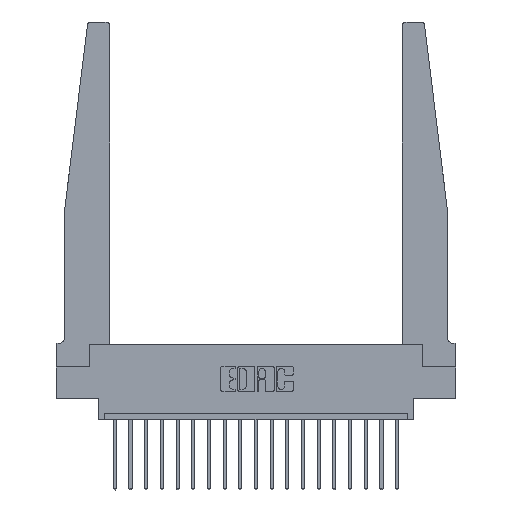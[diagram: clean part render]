
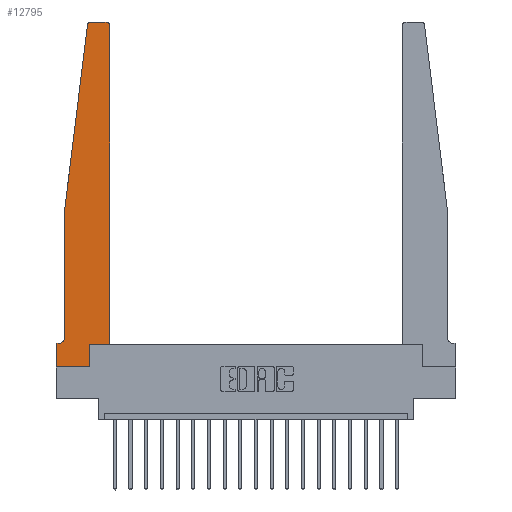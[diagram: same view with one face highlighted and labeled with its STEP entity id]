
A CAD part, top view. The second image highlights one B-rep face of the part: STEP entity #12795.
In plain terms, the highlighted planar face has unit normal (0, 0, 1).
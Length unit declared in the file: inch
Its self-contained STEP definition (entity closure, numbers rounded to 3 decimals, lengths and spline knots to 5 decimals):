
#38 = VECTOR ( 'NONE', #6142, 39.37008 ) ;
#186 = EDGE_CURVE ( 'NONE', #5363, #9330, #9167, .T. ) ;
#230 = EDGE_CURVE ( 'NONE', #16944, #18706, #1505, .T. ) ;
#235 = VECTOR ( 'NONE', #11786, 39.37008 ) ;
#839 = CARTESIAN_POINT ( 'NONE',  ( 0.2605, 0.18, 0.37 ) ) ;
#894 = DIRECTION ( 'NONE',  ( -0.122, -0.992, 0. ) ) ;
#999 = VERTEX_POINT ( 'NONE', #16890 ) ;
#1079 = EDGE_CURVE ( 'NONE', #7324, #6029, #4122, .T. ) ;
#1306 = CARTESIAN_POINT ( 'NONE',  ( 0., 0.1875, 0.37 ) ) ;
#1443 = DIRECTION ( 'NONE',  ( 1., 0., 0. ) ) ;
#1505 = LINE ( 'NONE', #12747, #19449 ) ;
#1701 = AXIS2_PLACEMENT_3D ( 'NONE', #11282, #2000, #12703 ) ;
#2000 = DIRECTION ( 'NONE',  ( 0., 0., -1. ) ) ;
#2064 = CIRCLE ( 'NONE', #1701, 0.05 ) ;
#2297 = CARTESIAN_POINT ( 'NONE',  ( 0.24675, 2.72367, 0.37 ) ) ;
#2537 = CARTESIAN_POINT ( 'NONE',  ( 0.2605, 0., 0.37 ) ) ;
#2604 = LINE ( 'NONE', #17732, #18651 ) ;
#2693 = ORIENTED_EDGE ( 'NONE', *, *, #6544, .T. ) ;
#2717 = VERTEX_POINT ( 'NONE', #5781 ) ;
#2848 = VERTEX_POINT ( 'NONE', #10034 ) ;
#2990 = EDGE_CURVE ( 'NONE', #15976, #16944, #7372, .T. ) ;
#3163 = EDGE_CURVE ( 'NONE', #2717, #12311, #14810, .T. ) ;
#3728 = CARTESIAN_POINT ( 'NONE',  ( 0.27653, 2.72, 0.37 ) ) ;
#3818 = LINE ( 'NONE', #16349, #235 ) ;
#4122 = LINE ( 'NONE', #18320, #38 ) ;
#4577 = PLANE ( 'NONE',  #9474 ) ;
#4659 = VECTOR ( 'NONE', #6564, 39.37008 ) ;
#4793 = CARTESIAN_POINT ( 'NONE',  ( 0.015, 0.1875, 0.37 ) ) ;
#5363 = VERTEX_POINT ( 'NONE', #4793 ) ;
#5781 = CARTESIAN_POINT ( 'NONE',  ( 0., 0., 0.37 ) ) ;
#6029 = VERTEX_POINT ( 'NONE', #18327 ) ;
#6142 = DIRECTION ( 'NONE',  ( 1., 0., 0. ) ) ;
#6544 = EDGE_CURVE ( 'NONE', #18706, #999, #19489, .T. ) ;
#6564 = DIRECTION ( 'NONE',  ( -1., 0., 0. ) ) ;
#6649 = CARTESIAN_POINT ( 'NONE',  ( 0., 0.1875, 0.37 ) ) ;
#6730 = DIRECTION ( 'NONE',  ( 0., 0., 1. ) ) ;
#6944 = CARTESIAN_POINT ( 'NONE',  ( 0.25, 2.75, 0.37 ) ) ;
#7072 = ORIENTED_EDGE ( 'NONE', *, *, #9172, .T. ) ;
#7324 = VERTEX_POINT ( 'NONE', #839 ) ;
#7372 = CIRCLE ( 'NONE', #12401, 0.03 ) ;
#7405 = ORIENTED_EDGE ( 'NONE', *, *, #2990, .T. ) ;
#8124 = DIRECTION ( 'NONE',  ( 1., 0., 0. ) ) ;
#8741 = DIRECTION ( 'NONE',  ( 0., 1., 0. ) ) ;
#9167 = LINE ( 'NONE', #18849, #4659 ) ;
#9172 = EDGE_CURVE ( 'NONE', #2848, #15976, #13660, .T. ) ;
#9330 = VERTEX_POINT ( 'NONE', #6649 ) ;
#9474 = AXIS2_PLACEMENT_3D ( 'NONE', #1306, #12198, #1443 ) ;
#9596 = VECTOR ( 'NONE', #11514, 39.37008 ) ;
#9600 = CARTESIAN_POINT ( 'NONE',  ( 0.395, 2.72, 0.37 ) ) ;
#9708 = AXIS2_PLACEMENT_3D ( 'NONE', #9600, #9785, #11363 ) ;
#9785 = DIRECTION ( 'NONE',  ( 0., 0., 1. ) ) ;
#9899 = CARTESIAN_POINT ( 'NONE',  ( 0.27653, 2.75, 0.37 ) ) ;
#10034 = CARTESIAN_POINT ( 'NONE',  ( 0.395, 2.75, 0.37 ) ) ;
#10244 = VECTOR ( 'NONE', #8124, 39.37008 ) ;
#10257 = ORIENTED_EDGE ( 'NONE', *, *, #18606, .T. ) ;
#10651 = FACE_OUTER_BOUND ( 'NONE', #11011, .T. ) ;
#10748 = EDGE_CURVE ( 'NONE', #9330, #2717, #2604, .T. ) ;
#10983 = VERTEX_POINT ( 'NONE', #14713 ) ;
#11011 = EDGE_LOOP ( 'NONE', ( #7072, #7405, #17081, #2693, #10257, #17054, #12189, #18938, #13365, #11149, #11372, #18903 ) ) ;
#11149 = ORIENTED_EDGE ( 'NONE', *, *, #1079, .T. ) ;
#11225 = CARTESIAN_POINT ( 'NONE',  ( 0., 0., 0.37 ) ) ;
#11282 = CARTESIAN_POINT ( 'NONE',  ( 0.015, 0.2375, 0.37 ) ) ;
#11363 = DIRECTION ( 'NONE',  ( 1., 0., 0. ) ) ;
#11372 = ORIENTED_EDGE ( 'NONE', *, *, #17017, .T. ) ;
#11514 = DIRECTION ( 'NONE',  ( -1., 0., 0. ) ) ;
#11786 = DIRECTION ( 'NONE',  ( 0., 1., 0. ) ) ;
#12189 = ORIENTED_EDGE ( 'NONE', *, *, #10748, .T. ) ;
#12198 = DIRECTION ( 'NONE',  ( 0., 0., 1. ) ) ;
#12311 = VERTEX_POINT ( 'NONE', #2537 ) ;
#12401 = AXIS2_PLACEMENT_3D ( 'NONE', #3728, #6730, #18752 ) ;
#12484 = EDGE_CURVE ( 'NONE', #10983, #2848, #17376, .T. ) ;
#12522 = VECTOR ( 'NONE', #8741, 39.37008 ) ;
#12703 = DIRECTION ( 'NONE',  ( -1., 0., 0. ) ) ;
#12747 = CARTESIAN_POINT ( 'NONE',  ( 0.065, 1.25, 0.37 ) ) ;
#12795 = ADVANCED_FACE ( 'NONE', ( #10651 ), #4577, .T. ) ;
#13365 = ORIENTED_EDGE ( 'NONE', *, *, #13941, .T. ) ;
#13660 = LINE ( 'NONE', #6944, #9596 ) ;
#13941 = EDGE_CURVE ( 'NONE', #12311, #7324, #19233, .T. ) ;
#14713 = CARTESIAN_POINT ( 'NONE',  ( 0.425, 2.72, 0.37 ) ) ;
#14810 = LINE ( 'NONE', #11225, #10244 ) ;
#15223 = CARTESIAN_POINT ( 'NONE',  ( 0.065, 1.25, 0.37 ) ) ;
#15976 = VERTEX_POINT ( 'NONE', #9899 ) ;
#16324 = DIRECTION ( 'NONE',  ( 0., -1., 0. ) ) ;
#16349 = CARTESIAN_POINT ( 'NONE',  ( 0.425, 0.18, 0.37 ) ) ;
#16367 = CARTESIAN_POINT ( 'NONE',  ( 0.2605, 0.18, 0.37 ) ) ;
#16863 = CARTESIAN_POINT ( 'NONE',  ( 0.065, 1.25, 0.37 ) ) ;
#16890 = CARTESIAN_POINT ( 'NONE',  ( 0.065, 0.2375, 0.37 ) ) ;
#16944 = VERTEX_POINT ( 'NONE', #2297 ) ;
#17017 = EDGE_CURVE ( 'NONE', #6029, #10983, #3818, .T. ) ;
#17054 = ORIENTED_EDGE ( 'NONE', *, *, #186, .T. ) ;
#17081 = ORIENTED_EDGE ( 'NONE', *, *, #230, .T. ) ;
#17343 = VECTOR ( 'NONE', #16324, 39.37008 ) ;
#17376 = CIRCLE ( 'NONE', #9708, 0.03 ) ;
#17671 = DIRECTION ( 'NONE',  ( 0., -1., 0. ) ) ;
#17732 = CARTESIAN_POINT ( 'NONE',  ( 0., 0., 0.37 ) ) ;
#18320 = CARTESIAN_POINT ( 'NONE',  ( 0.425, 0.18, 0.37 ) ) ;
#18327 = CARTESIAN_POINT ( 'NONE',  ( 0.425, 0.18, 0.37 ) ) ;
#18606 = EDGE_CURVE ( 'NONE', #999, #5363, #2064, .T. ) ;
#18651 = VECTOR ( 'NONE', #17671, 39.37008 ) ;
#18706 = VERTEX_POINT ( 'NONE', #16863 ) ;
#18752 = DIRECTION ( 'NONE',  ( 1., 0., 0. ) ) ;
#18849 = CARTESIAN_POINT ( 'NONE',  ( 0.065, 0.1875, 0.37 ) ) ;
#18903 = ORIENTED_EDGE ( 'NONE', *, *, #12484, .T. ) ;
#18938 = ORIENTED_EDGE ( 'NONE', *, *, #3163, .T. ) ;
#19233 = LINE ( 'NONE', #16367, #12522 ) ;
#19449 = VECTOR ( 'NONE', #894, 39.37008 ) ;
#19489 = LINE ( 'NONE', #15223, #17343 ) ;
